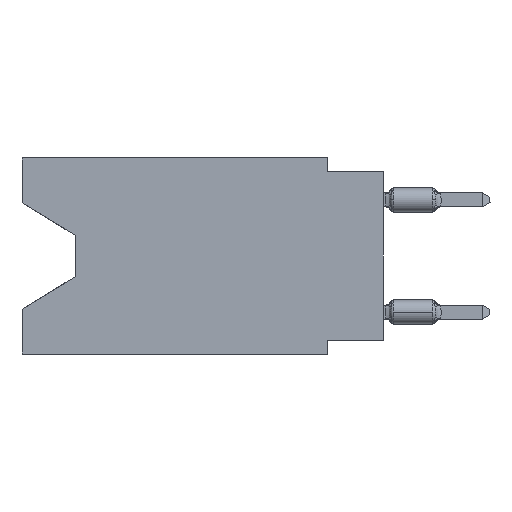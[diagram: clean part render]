
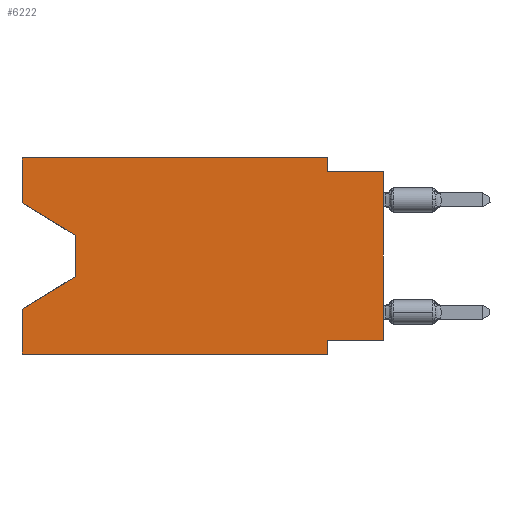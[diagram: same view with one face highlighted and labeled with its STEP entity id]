
A CAD part, left-side view. The second image highlights one B-rep face of the part: STEP entity #6222.
In plain terms, the highlighted planar face has unit normal (-1, 0, 0).
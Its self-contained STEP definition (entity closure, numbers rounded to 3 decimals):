
#62 = ORIENTED_EDGE ( 'NONE', *, *, #17966, .F. ) ;
#115 = EDGE_CURVE ( 'NONE', #21040, #7918, #23641, .T. ) ;
#427 = VECTOR ( 'NONE', #27562, 1000. ) ;
#1087 = VERTEX_POINT ( 'NONE', #22562 ) ;
#1233 = ORIENTED_EDGE ( 'NONE', *, *, #2975, .F. ) ;
#1277 = ORIENTED_EDGE ( 'NONE', *, *, #27817, .F. ) ;
#1545 = CARTESIAN_POINT ( 'NONE',  ( 0., 0., -0.635 ) ) ;
#1688 = LINE ( 'NONE', #1545, #19598 ) ;
#2280 = LINE ( 'NONE', #22385, #8516 ) ;
#2413 = ORIENTED_EDGE ( 'NONE', *, *, #115, .F. ) ;
#2769 = EDGE_CURVE ( 'NONE', #8624, #19087, #28186, .T. ) ;
#2975 = EDGE_CURVE ( 'NONE', #1087, #21040, #20406, .T. ) ;
#3065 = VERTEX_POINT ( 'NONE', #22801 ) ;
#3234 = CARTESIAN_POINT ( 'NONE',  ( 0., 2.54, 0. ) ) ;
#3829 = PLANE ( 'NONE',  #24715 ) ;
#4373 = LINE ( 'NONE', #20306, #18436 ) ;
#4504 = CARTESIAN_POINT ( 'NONE',  ( 0., 2.54, -8.89 ) ) ;
#4692 = ORIENTED_EDGE ( 'NONE', *, *, #10142, .T. ) ;
#5226 = CARTESIAN_POINT ( 'NONE',  ( 0., 0., 0. ) ) ;
#5703 = CARTESIAN_POINT ( 'NONE',  ( 0., 0., -8.255 ) ) ;
#6222 = ADVANCED_FACE ( 'NONE', ( #10555 ), #3829, .F. ) ;
#6532 = VECTOR ( 'NONE', #23568, 1000. ) ;
#6716 = ORIENTED_EDGE ( 'NONE', *, *, #2769, .F. ) ;
#6742 = DIRECTION ( 'NONE',  ( 0., -1., 0. ) ) ;
#7530 = CARTESIAN_POINT ( 'NONE',  ( 0., 0., -8.255 ) ) ;
#7833 = VECTOR ( 'NONE', #12325, 1000. ) ;
#7848 = EDGE_CURVE ( 'NONE', #3065, #1087, #10429, .T. ) ;
#7889 = DIRECTION ( 'NONE',  ( 0., 0., 1. ) ) ;
#7918 = VERTEX_POINT ( 'NONE', #25764 ) ;
#7923 = CARTESIAN_POINT ( 'NONE',  ( 0., 16.383, -6.852 ) ) ;
#8516 = VECTOR ( 'NONE', #6742, 1000. ) ;
#8580 = ORIENTED_EDGE ( 'NONE', *, *, #7848, .F. ) ;
#8624 = VERTEX_POINT ( 'NONE', #7530 ) ;
#9225 = VERTEX_POINT ( 'NONE', #15517 ) ;
#9647 = CARTESIAN_POINT ( 'NONE',  ( 0., 13.97, -3.505 ) ) ;
#10142 = EDGE_CURVE ( 'NONE', #22335, #22951, #4373, .T. ) ;
#10299 = ORIENTED_EDGE ( 'NONE', *, *, #23194, .T. ) ;
#10429 = LINE ( 'NONE', #12362, #13395 ) ;
#10526 = CARTESIAN_POINT ( 'NONE',  ( 0., 2.54, 0. ) ) ;
#10555 = FACE_OUTER_BOUND ( 'NONE', #22708, .T. ) ;
#10819 = VECTOR ( 'NONE', #17624, 1000. ) ;
#11099 = ORIENTED_EDGE ( 'NONE', *, *, #25039, .T. ) ;
#12325 = DIRECTION ( 'NONE',  ( 0., 0., -1. ) ) ;
#12362 = CARTESIAN_POINT ( 'NONE',  ( 0., 16.383, 0. ) ) ;
#13226 = CARTESIAN_POINT ( 'NONE',  ( 0., 13.97, -5.385 ) ) ;
#13395 = VECTOR ( 'NONE', #7889, 1000. ) ;
#13646 = EDGE_CURVE ( 'NONE', #9225, #22335, #13816, .T. ) ;
#13816 = LINE ( 'NONE', #9647, #27762 ) ;
#14292 = VERTEX_POINT ( 'NONE', #22388 ) ;
#15517 = CARTESIAN_POINT ( 'NONE',  ( 0., 13.97, -3.505 ) ) ;
#16916 = CARTESIAN_POINT ( 'NONE',  ( 0., 2.54, -8.255 ) ) ;
#17108 = DIRECTION ( 'NONE',  ( 1., 0., 0. ) ) ;
#17399 = CARTESIAN_POINT ( 'NONE',  ( 0., 16.383, 0. ) ) ;
#17624 = DIRECTION ( 'NONE',  ( 0., 0., 1. ) ) ;
#17732 = CARTESIAN_POINT ( 'NONE',  ( 0., 2.54, -8.89 ) ) ;
#17773 = LINE ( 'NONE', #4504, #18962 ) ;
#17966 = EDGE_CURVE ( 'NONE', #7918, #21812, #1688, .T. ) ;
#18062 = LINE ( 'NONE', #24611, #22771 ) ;
#18436 = VECTOR ( 'NONE', #23139, 1000. ) ;
#18962 = VECTOR ( 'NONE', #24465, 1000. ) ;
#19087 = VERTEX_POINT ( 'NONE', #16916 ) ;
#19476 = DIRECTION ( 'NONE',  ( 0., 0., -1. ) ) ;
#19598 = VECTOR ( 'NONE', #21804, 1000. ) ;
#19839 = VECTOR ( 'NONE', #20848, 1000. ) ;
#20256 = ORIENTED_EDGE ( 'NONE', *, *, #27851, .T. ) ;
#20306 = CARTESIAN_POINT ( 'NONE',  ( 0., 13.97, -5.385 ) ) ;
#20406 = LINE ( 'NONE', #25172, #19839 ) ;
#20440 = DIRECTION ( 'NONE',  ( 0., -0.855, -0.519 ) ) ;
#20848 = DIRECTION ( 'NONE',  ( 0., -1., 0. ) ) ;
#21040 = VERTEX_POINT ( 'NONE', #10526 ) ;
#21169 = ORIENTED_EDGE ( 'NONE', *, *, #13646, .T. ) ;
#21592 = EDGE_CURVE ( 'NONE', #14292, #22951, #21935, .T. ) ;
#21804 = DIRECTION ( 'NONE',  ( 0., -1., 0. ) ) ;
#21812 = VERTEX_POINT ( 'NONE', #23702 ) ;
#21935 = LINE ( 'NONE', #28791, #10819 ) ;
#21970 = VERTEX_POINT ( 'NONE', #17732 ) ;
#22335 = VERTEX_POINT ( 'NONE', #13226 ) ;
#22385 = CARTESIAN_POINT ( 'NONE',  ( 0., 16.383, -8.89 ) ) ;
#22388 = CARTESIAN_POINT ( 'NONE',  ( 0., 16.383, -8.89 ) ) ;
#22562 = CARTESIAN_POINT ( 'NONE',  ( 0., 16.383, 0. ) ) ;
#22708 = EDGE_LOOP ( 'NONE', ( #20256, #21169, #4692, #24061, #10299, #1277, #6716, #11099, #62, #2413, #1233, #8580 ) ) ;
#22754 = DIRECTION ( 'NONE',  ( 0., 0., -1. ) ) ;
#22771 = VECTOR ( 'NONE', #20440, 1000. ) ;
#22801 = CARTESIAN_POINT ( 'NONE',  ( 0., 16.383, -2.038 ) ) ;
#22951 = VERTEX_POINT ( 'NONE', #7923 ) ;
#23139 = DIRECTION ( 'NONE',  ( 0., 0.855, -0.519 ) ) ;
#23194 = EDGE_CURVE ( 'NONE', #14292, #21970, #2280, .T. ) ;
#23568 = DIRECTION ( 'NONE',  ( 0., 1., 0. ) ) ;
#23641 = LINE ( 'NONE', #3234, #7833 ) ;
#23702 = CARTESIAN_POINT ( 'NONE',  ( 0., 0., -0.635 ) ) ;
#24061 = ORIENTED_EDGE ( 'NONE', *, *, #21592, .F. ) ;
#24465 = DIRECTION ( 'NONE',  ( 0., 0., -1. ) ) ;
#24611 = CARTESIAN_POINT ( 'NONE',  ( 0., 16.383, -2.038 ) ) ;
#24715 = AXIS2_PLACEMENT_3D ( 'NONE', #17399, #17108, #19476 ) ;
#25039 = EDGE_CURVE ( 'NONE', #8624, #21812, #25622, .T. ) ;
#25172 = CARTESIAN_POINT ( 'NONE',  ( 0., 16.383, 0. ) ) ;
#25622 = LINE ( 'NONE', #5226, #427 ) ;
#25764 = CARTESIAN_POINT ( 'NONE',  ( 0., 2.54, -0.635 ) ) ;
#27562 = DIRECTION ( 'NONE',  ( 0., 0., 1. ) ) ;
#27762 = VECTOR ( 'NONE', #22754, 1000. ) ;
#27817 = EDGE_CURVE ( 'NONE', #19087, #21970, #17773, .T. ) ;
#27851 = EDGE_CURVE ( 'NONE', #3065, #9225, #18062, .T. ) ;
#28186 = LINE ( 'NONE', #5703, #6532 ) ;
#28791 = CARTESIAN_POINT ( 'NONE',  ( 0., 16.383, 0. ) ) ;
